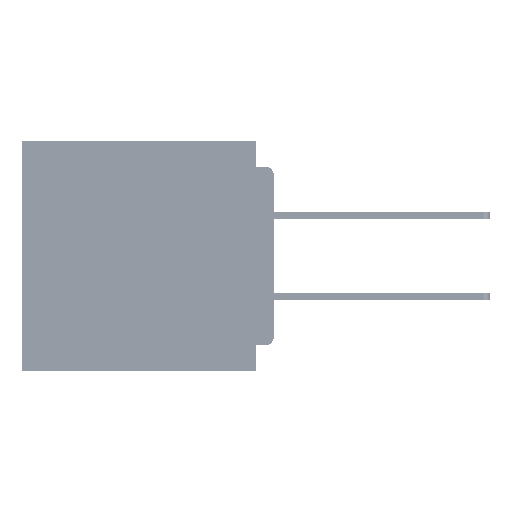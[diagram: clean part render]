
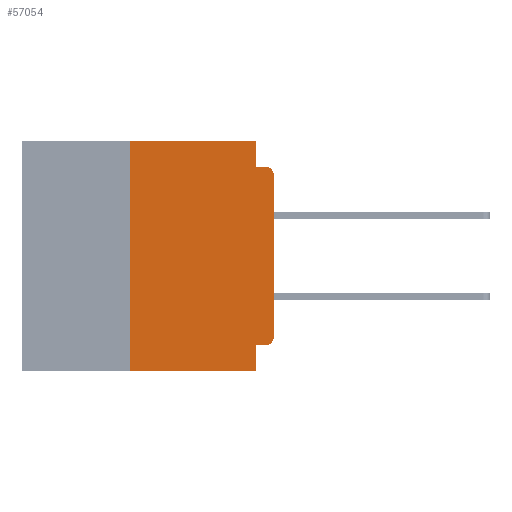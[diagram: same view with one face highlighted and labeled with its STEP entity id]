
A CAD part, left-side view. The second image highlights one B-rep face of the part: STEP entity #57054.
In plain terms, the highlighted planar face has unit normal (-1, 0, 0).
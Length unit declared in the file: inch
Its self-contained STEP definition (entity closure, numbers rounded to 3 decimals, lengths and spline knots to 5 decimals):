
#547 = CARTESIAN_POINT ( 'NONE',  ( 0., 0.031, -0.4 ) ) ;
#741 = DIRECTION ( 'NONE',  ( 0., -1., 0. ) ) ;
#1908 = VECTOR ( 'NONE', #741, 39.37008 ) ;
#1983 = LINE ( 'NONE', #53903, #60004 ) ;
#2023 = VECTOR ( 'NONE', #33018, 39.37008 ) ;
#3152 = EDGE_CURVE ( 'NONE', #66723, #16729, #64616, .T. ) ;
#4153 = CARTESIAN_POINT ( 'NONE',  ( 0., 0., -0.06 ) ) ;
#4351 = VERTEX_POINT ( 'NONE', #547 ) ;
#4937 = DIRECTION ( 'NONE',  ( -1., 0., 0. ) ) ;
#7051 = VECTOR ( 'NONE', #54747, 39.37008 ) ;
#7584 = EDGE_CURVE ( 'NONE', #11136, #28427, #33984, .T. ) ;
#8778 = LINE ( 'NONE', #49255, #7051 ) ;
#8988 = PLANE ( 'NONE',  #60259 ) ;
#9620 = ORIENTED_EDGE ( 'NONE', *, *, #14339, .F. ) ;
#9646 = VERTEX_POINT ( 'NONE', #4153 ) ;
#10974 = DIRECTION ( 'NONE',  ( -1., 0., 0. ) ) ;
#11034 = CARTESIAN_POINT ( 'NONE',  ( 0., 0.25, -0.4 ) ) ;
#11136 = VERTEX_POINT ( 'NONE', #66496 ) ;
#13249 = ORIENTED_EDGE ( 'NONE', *, *, #3152, .F. ) ;
#13789 = CARTESIAN_POINT ( 'NONE',  ( 0., 0., -0.045 ) ) ;
#13813 = ORIENTED_EDGE ( 'NONE', *, *, #15100, .T. ) ;
#14010 = ORIENTED_EDGE ( 'NONE', *, *, #18896, .F. ) ;
#14339 = EDGE_CURVE ( 'NONE', #16729, #4351, #1983, .T. ) ;
#14499 = CARTESIAN_POINT ( 'NONE',  ( 0., 0.031, 0. ) ) ;
#15100 = EDGE_CURVE ( 'NONE', #27289, #9646, #8778, .T. ) ;
#16729 = VERTEX_POINT ( 'NONE', #70180 ) ;
#18896 = EDGE_CURVE ( 'NONE', #66576, #42298, #45460, .T. ) ;
#19320 = CARTESIAN_POINT ( 'NONE',  ( 0., 0.015, -0.355 ) ) ;
#21315 = DIRECTION ( 'NONE',  ( 0., 0., -1. ) ) ;
#21531 = LINE ( 'NONE', #14499, #48747 ) ;
#22071 = EDGE_CURVE ( 'NONE', #66723, #27289, #42547, .T. ) ;
#23655 = ORIENTED_EDGE ( 'NONE', *, *, #31260, .F. ) ;
#24037 = CARTESIAN_POINT ( 'NONE',  ( 0., 0.437, -0.4 ) ) ;
#25449 = DIRECTION ( 'NONE',  ( 0., 0., -1. ) ) ;
#25860 = AXIS2_PLACEMENT_3D ( 'NONE', #37639, #4937, #43062 ) ;
#27289 = VERTEX_POINT ( 'NONE', #41790 ) ;
#28401 = DIRECTION ( 'NONE',  ( 0., 1., 0. ) ) ;
#28427 = VERTEX_POINT ( 'NONE', #63759 ) ;
#29111 = CARTESIAN_POINT ( 'NONE',  ( 0., 0.25, 0. ) ) ;
#29175 = CARTESIAN_POINT ( 'NONE',  ( 0., 0., -0.355 ) ) ;
#29531 = DIRECTION ( 'NONE',  ( 0., -1., 0. ) ) ;
#29744 = ORIENTED_EDGE ( 'NONE', *, *, #7584, .F. ) ;
#30367 = AXIS2_PLACEMENT_3D ( 'NONE', #43583, #10974, #49048 ) ;
#30950 = DIRECTION ( 'NONE',  ( 1., 0., 0. ) ) ;
#31260 = EDGE_CURVE ( 'NONE', #31762, #66576, #32843, .T. ) ;
#31762 = VERTEX_POINT ( 'NONE', #11034 ) ;
#32843 = LINE ( 'NONE', #49395, #2023 ) ;
#33018 = DIRECTION ( 'NONE',  ( 0., 0., 1. ) ) ;
#33984 = LINE ( 'NONE', #13789, #48433 ) ;
#33998 = VECTOR ( 'NONE', #28401, 39.37008 ) ;
#36198 = FACE_OUTER_BOUND ( 'NONE', #42877, .T. ) ;
#37639 = CARTESIAN_POINT ( 'NONE',  ( 0., 0.015, -0.34 ) ) ;
#39192 = ORIENTED_EDGE ( 'NONE', *, *, #47931, .F. ) ;
#40952 = LINE ( 'NONE', #24037, #53734 ) ;
#41325 = CIRCLE ( 'NONE', #30367, 0.015 ) ;
#41790 = CARTESIAN_POINT ( 'NONE',  ( 0., 0., -0.34 ) ) ;
#42298 = VERTEX_POINT ( 'NONE', #65142 ) ;
#42547 = CIRCLE ( 'NONE', #25860, 0.015 ) ;
#42877 = EDGE_LOOP ( 'NONE', ( #13813, #43096, #29744, #39192, #14010, #23655, #52083, #9620, #13249, #54699 ) ) ;
#43062 = DIRECTION ( 'NONE',  ( 0., 0., -1. ) ) ;
#43096 = ORIENTED_EDGE ( 'NONE', *, *, #52725, .T. ) ;
#43583 = CARTESIAN_POINT ( 'NONE',  ( 0., 0.015, -0.06 ) ) ;
#45460 = LINE ( 'NONE', #66036, #1908 ) ;
#46008 = EDGE_CURVE ( 'NONE', #31762, #4351, #40952, .T. ) ;
#47103 = CARTESIAN_POINT ( 'NONE',  ( 0., 0.437, 0. ) ) ;
#47931 = EDGE_CURVE ( 'NONE', #42298, #11136, #21531, .T. ) ;
#48433 = VECTOR ( 'NONE', #51875, 39.37008 ) ;
#48747 = VECTOR ( 'NONE', #25449, 39.37008 ) ;
#49048 = DIRECTION ( 'NONE',  ( 0., 0., -1. ) ) ;
#49255 = CARTESIAN_POINT ( 'NONE',  ( 0., 0., 0. ) ) ;
#49395 = CARTESIAN_POINT ( 'NONE',  ( 0., 0.25, -0.4 ) ) ;
#51875 = DIRECTION ( 'NONE',  ( 0., -1., 0. ) ) ;
#52083 = ORIENTED_EDGE ( 'NONE', *, *, #46008, .T. ) ;
#52725 = EDGE_CURVE ( 'NONE', #9646, #28427, #41325, .T. ) ;
#53734 = VECTOR ( 'NONE', #29531, 39.37008 ) ;
#53903 = CARTESIAN_POINT ( 'NONE',  ( 0., 0.031, -0.4 ) ) ;
#54699 = ORIENTED_EDGE ( 'NONE', *, *, #22071, .T. ) ;
#54747 = DIRECTION ( 'NONE',  ( 0., 0., 1. ) ) ;
#57054 = ADVANCED_FACE ( 'NONE', ( #36198 ), #8988, .F. ) ;
#60004 = VECTOR ( 'NONE', #21315, 39.37008 ) ;
#60259 = AXIS2_PLACEMENT_3D ( 'NONE', #47103, #30950, #68952 ) ;
#63759 = CARTESIAN_POINT ( 'NONE',  ( 0., 0.015, -0.045 ) ) ;
#64616 = LINE ( 'NONE', #29175, #33998 ) ;
#65142 = CARTESIAN_POINT ( 'NONE',  ( 0., 0.031, 0. ) ) ;
#66036 = CARTESIAN_POINT ( 'NONE',  ( 0., 0.437, 0. ) ) ;
#66496 = CARTESIAN_POINT ( 'NONE',  ( 0., 0.031, -0.045 ) ) ;
#66576 = VERTEX_POINT ( 'NONE', #29111 ) ;
#66723 = VERTEX_POINT ( 'NONE', #19320 ) ;
#68952 = DIRECTION ( 'NONE',  ( 0., 0., -1. ) ) ;
#70180 = CARTESIAN_POINT ( 'NONE',  ( 0., 0.031, -0.355 ) ) ;
